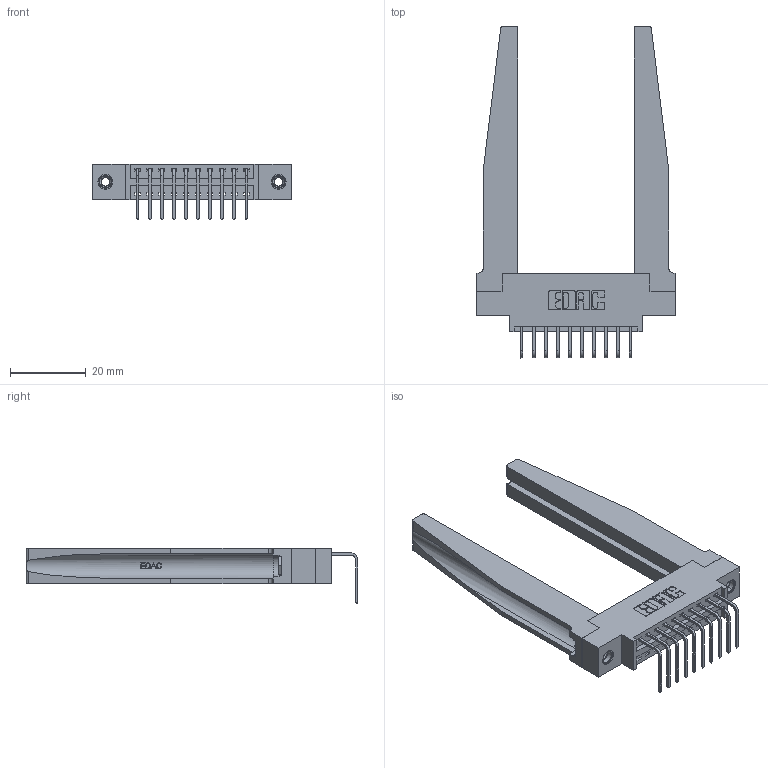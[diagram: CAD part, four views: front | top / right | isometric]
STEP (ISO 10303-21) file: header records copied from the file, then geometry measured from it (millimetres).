
FILE_DESCRIPTION (( 'STEP AP203' ), '1' );
FILE_NAME ('346-010-558-678.STEP', '2022-05-05T00:22:39', ( '' ), ( '' ), 'SwSTEP 2.0', 'SolidWorks 2020', '' );
FILE_SCHEMA (( 'CONFIG_CONTROL_DESIGN' ));
Length unit declared in the file: inch
Products named in the file (5): 345-292-001_558 Tail - 2; 346-220-078_345-220-078; 346-010-558-678; 345-250-001_345-250-001-102; 346 Part_0.170 Offset - 0.156 Dia-TH
Assembly tree (15 placements, depth 2):
  346-010-558-678
    346 Part_0.170 Offset - 0.156 Dia-TH
    345-292-001_558 Tail - 2  x10
    346-220-078_345-220-078  x2
    345-250-001_345-250-001-102  x2
Bounding box: 52.32 x 87.44 x 14.73 mm (x, y, z)
Volume: 11557.6 mm3; surface area: 12396.4 mm2
Topology: 15 solids, 15 shells, 974 faces, 2805 edges, 1846 vertices
Faces by surface type: plane 656, cylinder 266, bspline 36, cone 12, torus 4
Entity records: 15894 total; most frequent: CARTESIAN_POINT 3651, ORIENTED_EDGE 2482, DIRECTION 2243, EDGE_CURVE 1241, LINE 975, VECTOR 975, VERTEX_POINT 820, AXIS2_PLACEMENT_3D 634
